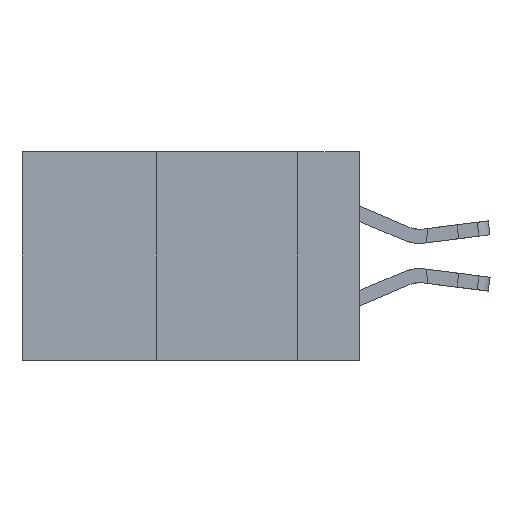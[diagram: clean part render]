
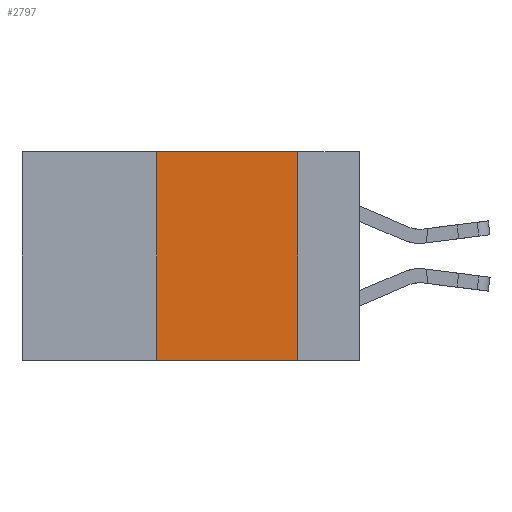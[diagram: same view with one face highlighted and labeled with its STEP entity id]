
A CAD part, left-side view. The second image highlights one B-rep face of the part: STEP entity #2797.
In plain terms, the highlighted planar face has unit normal (-1, 0, 0).
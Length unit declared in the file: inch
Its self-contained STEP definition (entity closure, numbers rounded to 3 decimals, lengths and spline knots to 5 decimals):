
#1105 = VECTOR ( 'NONE', #1619, 39.37008 ) ;
#1619 = DIRECTION ( 'NONE',  ( 0., 0., 1. ) ) ;
#1779 = CARTESIAN_POINT ( 'NONE',  ( 0., 0.11, 0. ) ) ;
#1937 = LINE ( 'NONE', #8504, #1105 ) ;
#2112 = FACE_OUTER_BOUND ( 'NONE', #10030, .T. ) ;
#2120 = DIRECTION ( 'NONE',  ( 0., 0., -1. ) ) ;
#2335 = DIRECTION ( 'NONE',  ( 0., -1., 0. ) ) ;
#2797 = ADVANCED_FACE ( 'NONE', ( #2112 ), #9244, .F. ) ;
#3132 = ORIENTED_EDGE ( 'NONE', *, *, #4376, .T. ) ;
#3296 = VECTOR ( 'NONE', #14156, 39.37008 ) ;
#4376 = EDGE_CURVE ( 'NONE', #8083, #15459, #13153, .T. ) ;
#4564 = ORIENTED_EDGE ( 'NONE', *, *, #21629, .F. ) ;
#4838 = ORIENTED_EDGE ( 'NONE', *, *, #19504, .F. ) ;
#5194 = CARTESIAN_POINT ( 'NONE',  ( 0., 0.6, -0.37 ) ) ;
#5267 = CARTESIAN_POINT ( 'NONE',  ( 0., 0.36, 0. ) ) ;
#5878 = CARTESIAN_POINT ( 'NONE',  ( 0., 0.11, 0. ) ) ;
#8083 = VERTEX_POINT ( 'NONE', #17780 ) ;
#8504 = CARTESIAN_POINT ( 'NONE',  ( 0., 0.36, 0. ) ) ;
#9244 = PLANE ( 'NONE',  #14954 ) ;
#10030 = EDGE_LOOP ( 'NONE', ( #4564, #4838, #19706, #3132 ) ) ;
#11059 = CARTESIAN_POINT ( 'NONE',  ( 0., 0.6, 0. ) ) ;
#11696 = EDGE_CURVE ( 'NONE', #8083, #12040, #1937, .T. ) ;
#11736 = CARTESIAN_POINT ( 'NONE',  ( 0., 0.11, -0.37 ) ) ;
#12040 = VERTEX_POINT ( 'NONE', #5267 ) ;
#12062 = VERTEX_POINT ( 'NONE', #5878 ) ;
#13153 = LINE ( 'NONE', #5194, #19080 ) ;
#14156 = DIRECTION ( 'NONE',  ( 0., 0., -1. ) ) ;
#14260 = DIRECTION ( 'NONE',  ( 1., 0., 0. ) ) ;
#14767 = VECTOR ( 'NONE', #2335, 39.37008 ) ;
#14954 = AXIS2_PLACEMENT_3D ( 'NONE', #11059, #14260, #2120 ) ;
#15288 = LINE ( 'NONE', #17903, #14767 ) ;
#15459 = VERTEX_POINT ( 'NONE', #11736 ) ;
#17447 = DIRECTION ( 'NONE',  ( 0., -1., 0. ) ) ;
#17780 = CARTESIAN_POINT ( 'NONE',  ( 0., 0.36, -0.37 ) ) ;
#17873 = LINE ( 'NONE', #1779, #3296 ) ;
#17903 = CARTESIAN_POINT ( 'NONE',  ( 0., 0.6, 0. ) ) ;
#19080 = VECTOR ( 'NONE', #17447, 39.37008 ) ;
#19504 = EDGE_CURVE ( 'NONE', #12040, #12062, #15288, .T. ) ;
#19706 = ORIENTED_EDGE ( 'NONE', *, *, #11696, .F. ) ;
#21629 = EDGE_CURVE ( 'NONE', #12062, #15459, #17873, .T. ) ;
